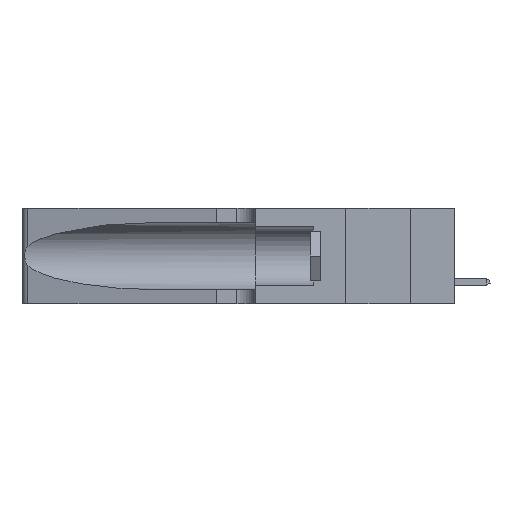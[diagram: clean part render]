
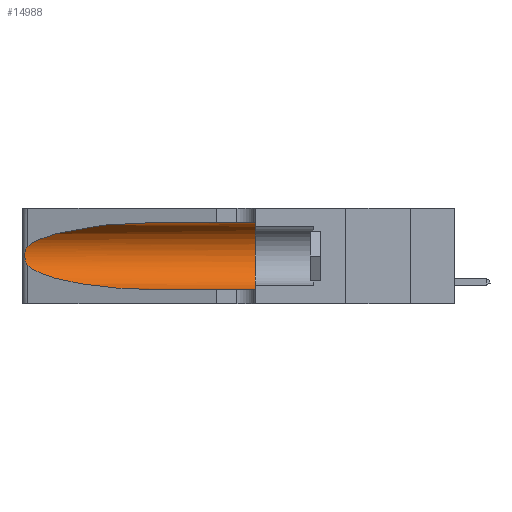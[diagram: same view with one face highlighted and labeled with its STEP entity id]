
A CAD part, left-side view. The second image highlights one B-rep face of the part: STEP entity #14988.
In plain terms, the highlighted cylindrical face has radius 3.308 mm (diameter 6.617 mm), a partial arc.
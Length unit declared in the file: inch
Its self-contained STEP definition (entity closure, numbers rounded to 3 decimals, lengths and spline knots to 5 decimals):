
#132 = VECTOR ( 'NONE', #26264, 39.37008 ) ;
#488 = CARTESIAN_POINT ( 'NONE',  ( 0.25639, 1.23186, 0.15144 ) ) ;
#890 = DIRECTION ( 'NONE',  ( 0., 0., -1. ) ) ;
#1149 = EDGE_CURVE ( 'NONE', #34291, #17670, #34853, .T. ) ;
#2215 = CARTESIAN_POINT ( 'NONE',  ( 0.1305, 1.61858, 0.05475 ) ) ;
#2422 = DIRECTION ( 'NONE',  ( 0., 1., 0. ) ) ;
#2611 = CARTESIAN_POINT ( 'NONE',  ( 0.25487, 1.22718, 0.22369 ) ) ;
#3227 = CARTESIAN_POINT ( 'NONE',  ( 0.25789, 1.23486, 0.15765 ) ) ;
#3395 = VERTEX_POINT ( 'NONE', #2611 ) ;
#3784 = CARTESIAN_POINT ( 'NONE',  ( 0.1305, 1.61858, 0.31525 ) ) ;
#4545 = ORIENTED_EDGE ( 'NONE', *, *, #1149, .F. ) ;
#4691 =( BOUNDED_CURVE ( )  B_SPLINE_CURVE ( 3, ( #8089, #13484, #21839, #27395 ),
 .UNSPECIFIED., .F., .F. ) 
 B_SPLINE_CURVE_WITH_KNOTS ( ( 4, 4 ),
 ( 1.5708, 2.84003 ),
 .UNSPECIFIED. ) 
 CURVE ( )  GEOMETRIC_REPRESENTATION_ITEM ( )  RATIONAL_B_SPLINE_CURVE ( ( 1., 0.87, 0.87, 1. ) ) 
 REPRESENTATION_ITEM ( '' )  );
#4942 = CARTESIAN_POINT ( 'NONE',  ( 0.25487, 1.22718, 0.14631 ) ) ;
#5726 = ORIENTED_EDGE ( 'NONE', *, *, #20509, .T. ) ;
#5930 = CARTESIAN_POINT ( 'NONE',  ( 0.26075, 1.23896, 0.178 ) ) ;
#6305 = LINE ( 'NONE', #3784, #132 ) ;
#7415 = B_SPLINE_CURVE_WITH_KNOTS ( 'NONE', 3,
 ( #32503, #35309, #32982, #27096, #24855, #19329, #33934, #5930, #13700, #17687, #3227, #488, #13174, #4942 ),
 .UNSPECIFIED., .F., .F.,
 ( 4, 2, 2, 2, 2, 2, 4 ),
 ( 0., 0.00027, 0.00053, 0.00107, 0.0016, 0.00187, 0.00214 ),
 .UNSPECIFIED. ) ;
#7802 = CARTESIAN_POINT ( 'NONE',  ( 0.25487, 1.22718, 0.14631 ) ) ;
#8076 = VERTEX_POINT ( 'NONE', #12731 ) ;
#8089 = CARTESIAN_POINT ( 'NONE',  ( 0.1305, 0.72297, 0.31525 ) ) ;
#9270 = DIRECTION ( 'NONE',  ( 0., -1., 0. ) ) ;
#9868 = VECTOR ( 'NONE', #35608, 39.37008 ) ;
#12003 = LINE ( 'NONE', #2215, #9868 ) ;
#12120 = CARTESIAN_POINT ( 'NONE',  ( 0.1305, 0.72297, 0.31525 ) ) ;
#12731 = CARTESIAN_POINT ( 'NONE',  ( 0.1305, 0.72297, 0.05475 ) ) ;
#13174 = CARTESIAN_POINT ( 'NONE',  ( 0.25555, 1.22993, 0.14849 ) ) ;
#13484 = CARTESIAN_POINT ( 'NONE',  ( 0.18966, 0.96281, 0.31525 ) ) ;
#13573 = CARTESIAN_POINT ( 'NONE',  ( 0.2373, 1.15595, 0.08982 ) ) ;
#13700 = CARTESIAN_POINT ( 'NONE',  ( 0.26017, 1.23833, 0.17102 ) ) ;
#13928 = CARTESIAN_POINT ( 'NONE',  ( 0.1305, 0.72297, 0.05475 ) ) ;
#14313 = EDGE_CURVE ( 'NONE', #33510, #8076, #30182, .T. ) ;
#14371 = EDGE_CURVE ( 'NONE', #3395, #33510, #7415, .T. ) ;
#14988 = ADVANCED_FACE ( 'NONE', ( #29254 ), #32788, .F. ) ;
#15682 = CARTESIAN_POINT ( 'NONE',  ( 0.1305, 0.35, 0.31525 ) ) ;
#16806 = ORIENTED_EDGE ( 'NONE', *, *, #31184, .F. ) ;
#17670 = VERTEX_POINT ( 'NONE', #20782 ) ;
#17687 = CARTESIAN_POINT ( 'NONE',  ( 0.25856, 1.23593, 0.16098 ) ) ;
#18706 = VERTEX_POINT ( 'NONE', #12120 ) ;
#19219 = CARTESIAN_POINT ( 'NONE',  ( 0.1305, 0.35, 0.185 ) ) ;
#19329 = CARTESIAN_POINT ( 'NONE',  ( 0.26018, 1.23835, 0.19895 ) ) ;
#20509 = EDGE_CURVE ( 'NONE', #8076, #17670, #12003, .T. ) ;
#20782 = CARTESIAN_POINT ( 'NONE',  ( 0.1305, 0.35, 0.05475 ) ) ;
#21839 = CARTESIAN_POINT ( 'NONE',  ( 0.2373, 1.15595, 0.28018 ) ) ;
#22751 = ORIENTED_EDGE ( 'NONE', *, *, #14371, .T. ) ;
#22801 = AXIS2_PLACEMENT_3D ( 'NONE', #26082, #9270, #890 ) ;
#24855 = CARTESIAN_POINT ( 'NONE',  ( 0.25854, 1.2359, 0.20912 ) ) ;
#25111 = CARTESIAN_POINT ( 'NONE',  ( 0.18966, 0.96281, 0.05475 ) ) ;
#26082 = CARTESIAN_POINT ( 'NONE',  ( 0.1305, 1.61858, 0.185 ) ) ;
#26264 = DIRECTION ( 'NONE',  ( 0., -1., 0. ) ) ;
#26960 = EDGE_LOOP ( 'NONE', ( #33375, #22751, #31248, #5726, #4545, #16806 ) ) ;
#27096 = CARTESIAN_POINT ( 'NONE',  ( 0.25787, 1.23484, 0.2124 ) ) ;
#27395 = CARTESIAN_POINT ( 'NONE',  ( 0.25487, 1.22718, 0.22369 ) ) ;
#27827 = DIRECTION ( 'NONE',  ( 0., 0., 1. ) ) ;
#29254 = FACE_OUTER_BOUND ( 'NONE', #26960, .T. ) ;
#29337 = AXIS2_PLACEMENT_3D ( 'NONE', #19219, #2422, #27827 ) ;
#30182 =( BOUNDED_CURVE ( )  B_SPLINE_CURVE ( 3, ( #7802, #13573, #25111, #13928 ),
 .UNSPECIFIED., .F., .T. ) 
 B_SPLINE_CURVE_WITH_KNOTS ( ( 4, 4 ),
 ( 3.44316, 4.71239 ),
 .UNSPECIFIED. ) 
 CURVE ( )  GEOMETRIC_REPRESENTATION_ITEM ( )  RATIONAL_B_SPLINE_CURVE ( ( 1., 0.87, 0.87, 1. ) ) 
 REPRESENTATION_ITEM ( '' )  );
#31184 = EDGE_CURVE ( 'NONE', #18706, #34291, #6305, .T. ) ;
#31248 = ORIENTED_EDGE ( 'NONE', *, *, #14313, .T. ) ;
#31366 = EDGE_CURVE ( 'NONE', #18706, #3395, #4691, .T. ) ;
#32503 = CARTESIAN_POINT ( 'NONE',  ( 0.25487, 1.22718, 0.22369 ) ) ;
#32788 = CYLINDRICAL_SURFACE ( 'NONE', #22801, 0.13025 ) ;
#32982 = CARTESIAN_POINT ( 'NONE',  ( 0.25639, 1.23184, 0.21858 ) ) ;
#33375 = ORIENTED_EDGE ( 'NONE', *, *, #31366, .T. ) ;
#33510 = VERTEX_POINT ( 'NONE', #34041 ) ;
#33934 = CARTESIAN_POINT ( 'NONE',  ( 0.26075, 1.23896, 0.19203 ) ) ;
#34041 = CARTESIAN_POINT ( 'NONE',  ( 0.25487, 1.22718, 0.14631 ) ) ;
#34291 = VERTEX_POINT ( 'NONE', #15682 ) ;
#34853 = CIRCLE ( 'NONE', #29337, 0.13025 ) ;
#35309 = CARTESIAN_POINT ( 'NONE',  ( 0.25555, 1.22994, 0.2215 ) ) ;
#35608 = DIRECTION ( 'NONE',  ( 0., -1., 0. ) ) ;
